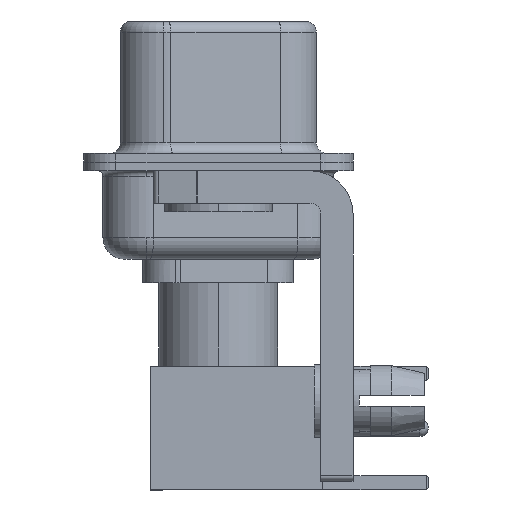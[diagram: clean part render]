
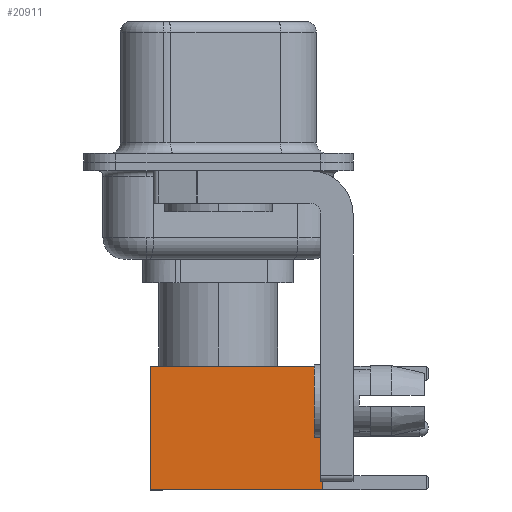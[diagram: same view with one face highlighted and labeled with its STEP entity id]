
A CAD part, left-side view. The second image highlights one B-rep face of the part: STEP entity #20911.
In plain terms, the highlighted face is planar.
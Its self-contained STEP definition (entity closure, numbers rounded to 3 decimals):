
#52 = ORIENTED_EDGE ( 'NONE', *, *, #13066, .F. ) ;
#1028 = VECTOR ( 'NONE', #19079, 1000. ) ;
#1070 = EDGE_CURVE ( 'NONE', #10008, #16867, #9162, .T. ) ;
#1498 = ORIENTED_EDGE ( 'NONE', *, *, #1070, .F. ) ;
#2998 = EDGE_LOOP ( 'NONE', ( #9003, #10409, #1498, #52 ) ) ;
#3211 = CARTESIAN_POINT ( 'NONE',  ( 2.875, 2.875, 8. ) ) ;
#4304 = CARTESIAN_POINT ( 'NONE',  ( 2.875, 2.875, 0. ) ) ;
#4661 = EDGE_CURVE ( 'NONE', #16316, #16867, #23068, .T. ) ;
#5452 = EDGE_CURVE ( 'NONE', #18967, #16316, #14825, .T. ) ;
#5460 = CARTESIAN_POINT ( 'NONE',  ( 0., 2.875, 8. ) ) ;
#6291 = FACE_OUTER_BOUND ( 'NONE', #2998, .T. ) ;
#7684 = DIRECTION ( 'NONE',  ( 0., 0., -1. ) ) ;
#8296 = PLANE ( 'NONE',  #19669 ) ;
#8650 = DIRECTION ( 'NONE',  ( 0., 0., 1. ) ) ;
#9003 = ORIENTED_EDGE ( 'NONE', *, *, #5452, .T. ) ;
#9162 = LINE ( 'NONE', #11269, #14629 ) ;
#10008 = VERTEX_POINT ( 'NONE', #10947 ) ;
#10409 = ORIENTED_EDGE ( 'NONE', *, *, #4661, .T. ) ;
#10947 = CARTESIAN_POINT ( 'NONE',  ( -2.875, 2.875, 8. ) ) ;
#11269 = CARTESIAN_POINT ( 'NONE',  ( -2.875, 2.875, 0. ) ) ;
#11564 = LINE ( 'NONE', #5460, #22742 ) ;
#13066 = EDGE_CURVE ( 'NONE', #18967, #10008, #11564, .T. ) ;
#13178 = DIRECTION ( 'NONE',  ( -1., 0., 0. ) ) ;
#13197 = CARTESIAN_POINT ( 'NONE',  ( -2.875, 2.875, 0. ) ) ;
#14629 = VECTOR ( 'NONE', #7684, 1000. ) ;
#14825 = LINE ( 'NONE', #16953, #1028 ) ;
#14965 = CARTESIAN_POINT ( 'NONE',  ( 2.875, 2.875, 0. ) ) ;
#15456 = CARTESIAN_POINT ( 'NONE',  ( 0., 2.875, 0. ) ) ;
#16116 = VECTOR ( 'NONE', #18841, 1000. ) ;
#16316 = VERTEX_POINT ( 'NONE', #14965 ) ;
#16867 = VERTEX_POINT ( 'NONE', #13197 ) ;
#16953 = CARTESIAN_POINT ( 'NONE',  ( 2.875, 2.875, 0. ) ) ;
#18841 = DIRECTION ( 'NONE',  ( -1., 0., 0. ) ) ;
#18967 = VERTEX_POINT ( 'NONE', #3211 ) ;
#19079 = DIRECTION ( 'NONE',  ( 0., 0., -1. ) ) ;
#19669 = AXIS2_PLACEMENT_3D ( 'NONE', #4304, #19986, #8650 ) ;
#19986 = DIRECTION ( 'NONE',  ( 0., 1., 0. ) ) ;
#20911 = ADVANCED_FACE ( 'NONE', ( #6291 ), #8296, .T. ) ;
#22742 = VECTOR ( 'NONE', #13178, 1000. ) ;
#23068 = LINE ( 'NONE', #15456, #16116 ) ;
